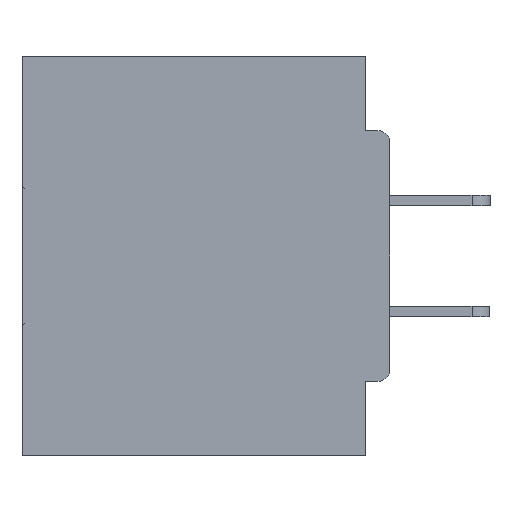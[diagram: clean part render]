
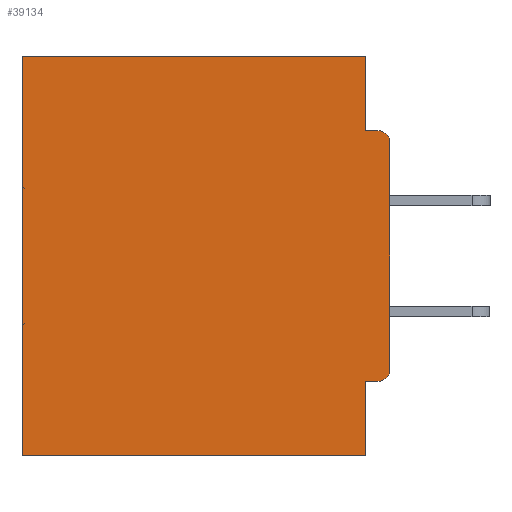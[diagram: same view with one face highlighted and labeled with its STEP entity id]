
A CAD part, left-side view. The second image highlights one B-rep face of the part: STEP entity #39134.
In plain terms, the highlighted planar face has unit normal (-1, 0, 0).
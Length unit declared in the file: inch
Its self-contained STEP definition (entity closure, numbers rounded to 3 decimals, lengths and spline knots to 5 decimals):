
#772 = LINE ( 'NONE', #40704, #25209 ) ;
#1476 = VECTOR ( 'NONE', #24883, 39.37008 ) ;
#2091 = VERTEX_POINT ( 'NONE', #4684 ) ;
#2185 = CARTESIAN_POINT ( 'NONE',  ( 0.298, 0.031, -0.5 ) ) ;
#2799 = LINE ( 'NONE', #35613, #11206 ) ;
#3556 = CARTESIAN_POINT ( 'NONE',  ( 0.298, 0.46, 0. ) ) ;
#3747 = DIRECTION ( 'NONE',  ( 0., 1., 0. ) ) ;
#4376 = CIRCLE ( 'NONE', #22415, 0.015 ) ;
#4684 = CARTESIAN_POINT ( 'NONE',  ( 0.298, 0.46, -0.5 ) ) ;
#5043 = CARTESIAN_POINT ( 'NONE',  ( 0.298, 0., 0. ) ) ;
#5710 = EDGE_CURVE ( 'NONE', #7869, #8320, #32698, .T. ) ;
#6298 = CARTESIAN_POINT ( 'NONE',  ( 0.298, 0.031, -0.5 ) ) ;
#7415 = CARTESIAN_POINT ( 'NONE',  ( 0.298, 0., -0.0935 ) ) ;
#7769 = EDGE_CURVE ( 'NONE', #42219, #42419, #772, .T. ) ;
#7869 = VERTEX_POINT ( 'NONE', #20757 ) ;
#8320 = VERTEX_POINT ( 'NONE', #36941 ) ;
#8619 = EDGE_CURVE ( 'NONE', #27636, #2091, #9572, .T. ) ;
#8688 = VERTEX_POINT ( 'NONE', #13643 ) ;
#9572 = LINE ( 'NONE', #3556, #32971 ) ;
#9853 = CARTESIAN_POINT ( 'NONE',  ( 0.298, 0.46, 0. ) ) ;
#10544 = VECTOR ( 'NONE', #11254, 39.37008 ) ;
#10970 = VECTOR ( 'NONE', #16180, 39.37008 ) ;
#11032 = CARTESIAN_POINT ( 'NONE',  ( 0.298, 0.015, -0.4065 ) ) ;
#11206 = VECTOR ( 'NONE', #15708, 39.37008 ) ;
#11254 = DIRECTION ( 'NONE',  ( 0., -1., 0. ) ) ;
#11364 = ORIENTED_EDGE ( 'NONE', *, *, #40364, .T. ) ;
#11775 = DIRECTION ( 'NONE',  ( -1., 0., 0. ) ) ;
#12064 = PLANE ( 'NONE',  #37716 ) ;
#12349 = CARTESIAN_POINT ( 'NONE',  ( 0.298, 0.031, 0. ) ) ;
#12460 = ORIENTED_EDGE ( 'NONE', *, *, #29451, .F. ) ;
#13643 = CARTESIAN_POINT ( 'NONE',  ( 0.298, 0.031, -0.0935 ) ) ;
#14487 = DIRECTION ( 'NONE',  ( 0., 0., -1. ) ) ;
#14836 = VERTEX_POINT ( 'NONE', #2185 ) ;
#14928 = VECTOR ( 'NONE', #38281, 39.37008 ) ;
#15266 = DIRECTION ( 'NONE',  ( 0., 0., -1. ) ) ;
#15546 = CARTESIAN_POINT ( 'NONE',  ( 0.298, 0.015, -0.0935 ) ) ;
#15708 = DIRECTION ( 'NONE',  ( 0., 1., 0. ) ) ;
#16180 = DIRECTION ( 'NONE',  ( 0., 1., 0. ) ) ;
#19161 = AXIS2_PLACEMENT_3D ( 'NONE', #31673, #11775, #15266 ) ;
#19232 = EDGE_CURVE ( 'NONE', #42419, #14836, #36802, .T. ) ;
#20304 = LINE ( 'NONE', #39324, #10970 ) ;
#20753 = CARTESIAN_POINT ( 'NONE',  ( 0.298, 0.031, -0.4065 ) ) ;
#20757 = CARTESIAN_POINT ( 'NONE',  ( 0.298, 0., -0.1085 ) ) ;
#21591 = ORIENTED_EDGE ( 'NONE', *, *, #26110, .T. ) ;
#21683 = VECTOR ( 'NONE', #32209, 39.37008 ) ;
#22415 = AXIS2_PLACEMENT_3D ( 'NONE', #30568, #34655, #14487 ) ;
#23159 = EDGE_CURVE ( 'NONE', #42219, #8320, #25970, .T. ) ;
#24234 = LINE ( 'NONE', #34363, #14928 ) ;
#24883 = DIRECTION ( 'NONE',  ( 0., 0., -1. ) ) ;
#25209 = VECTOR ( 'NONE', #3747, 39.37008 ) ;
#25970 = CIRCLE ( 'NONE', #19161, 0.015 ) ;
#26090 = ORIENTED_EDGE ( 'NONE', *, *, #38201, .F. ) ;
#26110 = EDGE_CURVE ( 'NONE', #32779, #27636, #2799, .T. ) ;
#27636 = VERTEX_POINT ( 'NONE', #9853 ) ;
#28050 = ORIENTED_EDGE ( 'NONE', *, *, #23159, .T. ) ;
#29265 = LINE ( 'NONE', #7415, #10544 ) ;
#29451 = EDGE_CURVE ( 'NONE', #8688, #37632, #29265, .T. ) ;
#29496 = ORIENTED_EDGE ( 'NONE', *, *, #19232, .F. ) ;
#30568 = CARTESIAN_POINT ( 'NONE',  ( 0.298, 0.015, -0.1085 ) ) ;
#30572 = EDGE_CURVE ( 'NONE', #14836, #2091, #20304, .T. ) ;
#31673 = CARTESIAN_POINT ( 'NONE',  ( 0.298, 0.015, -0.3915 ) ) ;
#31815 = EDGE_LOOP ( 'NONE', ( #11364, #12460, #26090, #21591, #39628, #34208, #29496, #32623, #28050, #36348 ) ) ;
#32209 = DIRECTION ( 'NONE',  ( 0., 0., -1. ) ) ;
#32623 = ORIENTED_EDGE ( 'NONE', *, *, #7769, .F. ) ;
#32698 = LINE ( 'NONE', #41397, #1476 ) ;
#32779 = VERTEX_POINT ( 'NONE', #12349 ) ;
#32971 = VECTOR ( 'NONE', #43014, 39.37008 ) ;
#34208 = ORIENTED_EDGE ( 'NONE', *, *, #30572, .F. ) ;
#34363 = CARTESIAN_POINT ( 'NONE',  ( 0.298, 0.031, -0.5 ) ) ;
#34655 = DIRECTION ( 'NONE',  ( -1., 0., 0. ) ) ;
#35325 = DIRECTION ( 'NONE',  ( 0., 0., -1. ) ) ;
#35613 = CARTESIAN_POINT ( 'NONE',  ( 0.298, 0., 0. ) ) ;
#36348 = ORIENTED_EDGE ( 'NONE', *, *, #5710, .F. ) ;
#36802 = LINE ( 'NONE', #6298, #21683 ) ;
#36941 = CARTESIAN_POINT ( 'NONE',  ( 0.298, 0., -0.3915 ) ) ;
#37632 = VERTEX_POINT ( 'NONE', #15546 ) ;
#37716 = AXIS2_PLACEMENT_3D ( 'NONE', #5043, #42159, #35325 ) ;
#38201 = EDGE_CURVE ( 'NONE', #32779, #8688, #24234, .T. ) ;
#38281 = DIRECTION ( 'NONE',  ( 0., 0., -1. ) ) ;
#39134 = ADVANCED_FACE ( 'NONE', ( #42402 ), #12064, .F. ) ;
#39324 = CARTESIAN_POINT ( 'NONE',  ( 0.298, 0., -0.5 ) ) ;
#39628 = ORIENTED_EDGE ( 'NONE', *, *, #8619, .T. ) ;
#40364 = EDGE_CURVE ( 'NONE', #7869, #37632, #4376, .T. ) ;
#40704 = CARTESIAN_POINT ( 'NONE',  ( 0.298, 0., -0.4065 ) ) ;
#41397 = CARTESIAN_POINT ( 'NONE',  ( 0.298, 0., 0. ) ) ;
#42159 = DIRECTION ( 'NONE',  ( 1., 0., 0. ) ) ;
#42219 = VERTEX_POINT ( 'NONE', #11032 ) ;
#42402 = FACE_OUTER_BOUND ( 'NONE', #31815, .T. ) ;
#42419 = VERTEX_POINT ( 'NONE', #20753 ) ;
#43014 = DIRECTION ( 'NONE',  ( 0., 0., -1. ) ) ;
